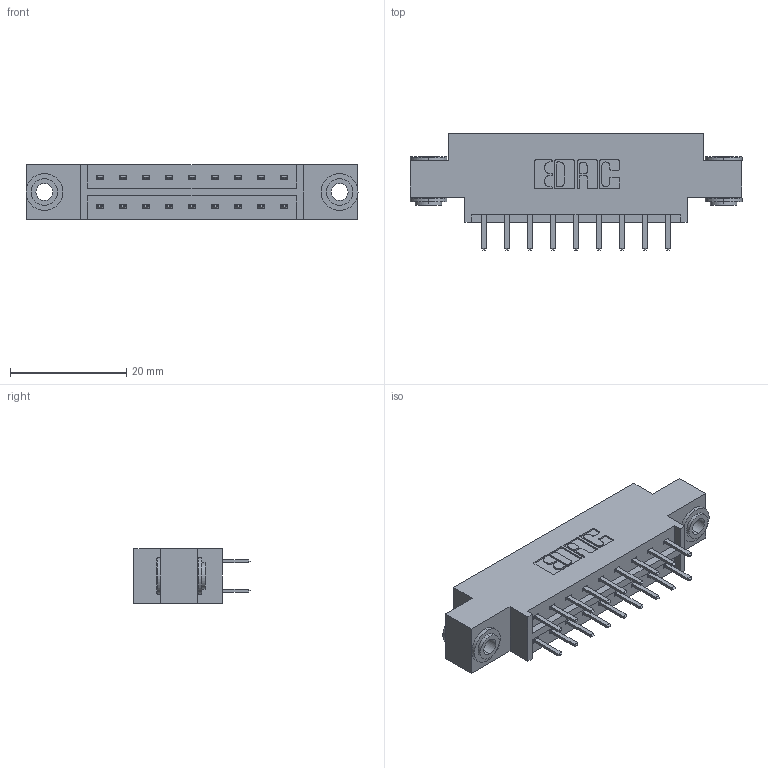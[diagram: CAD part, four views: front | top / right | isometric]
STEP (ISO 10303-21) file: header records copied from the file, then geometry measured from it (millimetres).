
FILE_DESCRIPTION (( 'STEP AP203' ), '1' );
FILE_NAME ('333-018-520-803.STEP', '2019-08-09T12:44:46', ( '' ), ( '' ), 'SwSTEP 2.0', 'SolidWorks 2016', '' );
FILE_SCHEMA (( 'CONFIG_CONTROL_DESIGN' ));
Length unit declared in the file: inch
Products named in the file (4): 333 Part_Offset - .156 Dia - TH; 333-018-520-803; 345-250-002_345-250-002-102; 345-292-001_345-293-120
Assembly tree (21 placements, depth 2):
  333-018-520-803
    333 Part_Offset - .156 Dia - TH
    345-292-001_345-293-120  x18
    345-250-002_345-250-002-102  x2
Bounding box: 57.2 x 20.02 x 9.4 mm (x, y, z)
Volume: 5315 mm3; surface area: 6349.8 mm2
Topology: 21 solids, 21 shells, 1164 faces, 3333 edges, 2170 vertices
Faces by surface type: plane 768, cylinder 388, cone 8
Entity records: 10954 total; most frequent: CARTESIAN_POINT 1845, ORIENTED_EDGE 1762, DIRECTION 1655, EDGE_CURVE 881, LINE 725, VECTOR 725, VERTEX_POINT 582, AXIS2_PLACEMENT_3D 465
